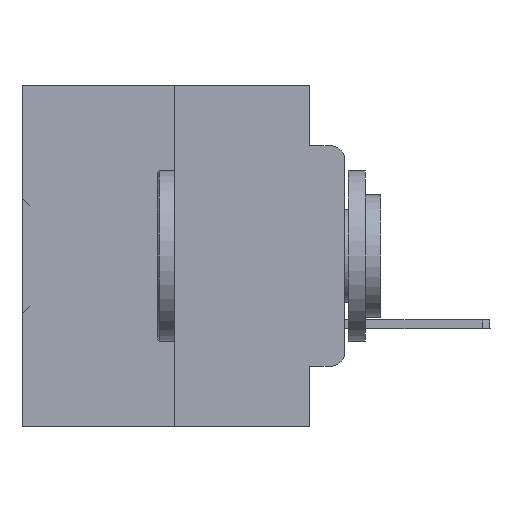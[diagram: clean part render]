
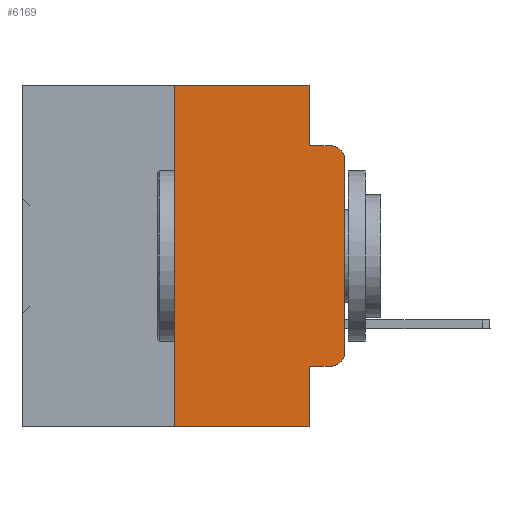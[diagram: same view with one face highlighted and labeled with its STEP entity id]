
A CAD part, left-side view. The second image highlights one B-rep face of the part: STEP entity #6169.
In plain terms, the highlighted planar face has unit normal (-1, 0, 0).
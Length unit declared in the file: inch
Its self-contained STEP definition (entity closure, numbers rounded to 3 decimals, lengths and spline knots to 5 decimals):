
#433 = EDGE_CURVE ( 'NONE', #15531, #33314, #8550, .T. ) ;
#893 = EDGE_CURVE ( 'NONE', #14730, #23608, #2235, .T. ) ;
#1037 = DIRECTION ( 'NONE',  ( -1., 0., 0. ) ) ;
#1055 = CARTESIAN_POINT ( 'NONE',  ( 0., 0.02, -0.4115 ) ) ;
#1373 = EDGE_CURVE ( 'NONE', #15531, #6546, #26735, .T. ) ;
#2119 = DIRECTION ( 'NONE',  ( 0., 0., -1. ) ) ;
#2175 = EDGE_CURVE ( 'NONE', #32285, #13042, #3916, .T. ) ;
#2187 = CIRCLE ( 'NONE', #2769, 0.02 ) ;
#2235 = LINE ( 'NONE', #36081, #32246 ) ;
#2302 = EDGE_CURVE ( 'NONE', #16048, #32285, #34897, .T. ) ;
#2687 = CARTESIAN_POINT ( 'NONE',  ( 0., 0.02, -0.0885 ) ) ;
#2769 = AXIS2_PLACEMENT_3D ( 'NONE', #16671, #11611, #9258 ) ;
#3916 = CIRCLE ( 'NONE', #25714, 0.02 ) ;
#4508 = ORIENTED_EDGE ( 'NONE', *, *, #27720, .T. ) ;
#6000 = ORIENTED_EDGE ( 'NONE', *, *, #433, .F. ) ;
#6111 = ORIENTED_EDGE ( 'NONE', *, *, #1373, .T. ) ;
#6169 = ADVANCED_FACE ( 'NONE', ( #13378 ), #34118, .F. ) ;
#6546 = VERTEX_POINT ( 'NONE', #1055 ) ;
#8550 = LINE ( 'NONE', #13846, #23174 ) ;
#8713 = VECTOR ( 'NONE', #26319, 39.37008 ) ;
#9154 = CARTESIAN_POINT ( 'NONE',  ( 0., 0., -0.1085 ) ) ;
#9258 = DIRECTION ( 'NONE',  ( 0., 0., -1. ) ) ;
#9400 = VERTEX_POINT ( 'NONE', #15428 ) ;
#9628 = ORIENTED_EDGE ( 'NONE', *, *, #30023, .F. ) ;
#10316 = CARTESIAN_POINT ( 'NONE',  ( 0., 0.051, 0. ) ) ;
#11221 = CARTESIAN_POINT ( 'NONE',  ( 0., 0., 0. ) ) ;
#11611 = DIRECTION ( 'NONE',  ( -1., 0., 0. ) ) ;
#12329 = LINE ( 'NONE', #17293, #8713 ) ;
#13042 = VERTEX_POINT ( 'NONE', #2687 ) ;
#13378 = FACE_OUTER_BOUND ( 'NONE', #24268, .T. ) ;
#13846 = CARTESIAN_POINT ( 'NONE',  ( 0., 0.051, 0. ) ) ;
#14137 = DIRECTION ( 'NONE',  ( 0., 0., 1. ) ) ;
#14222 = ORIENTED_EDGE ( 'NONE', *, *, #893, .F. ) ;
#14730 = VERTEX_POINT ( 'NONE', #10316 ) ;
#15428 = CARTESIAN_POINT ( 'NONE',  ( 0., 0.25, 0. ) ) ;
#15531 = VERTEX_POINT ( 'NONE', #16710 ) ;
#16048 = VERTEX_POINT ( 'NONE', #23652 ) ;
#16671 = CARTESIAN_POINT ( 'NONE',  ( 0., 0.02, -0.3915 ) ) ;
#16710 = CARTESIAN_POINT ( 'NONE',  ( 0., 0.051, -0.4115 ) ) ;
#16753 = VECTOR ( 'NONE', #24109, 39.37008 ) ;
#17137 = DIRECTION ( 'NONE',  ( 0., -1., 0. ) ) ;
#17293 = CARTESIAN_POINT ( 'NONE',  ( 0., 0.051, -0.0885 ) ) ;
#17766 = ORIENTED_EDGE ( 'NONE', *, *, #2175, .T. ) ;
#17842 = ORIENTED_EDGE ( 'NONE', *, *, #27552, .T. ) ;
#18641 = DIRECTION ( 'NONE',  ( 0., 0., -1. ) ) ;
#20095 = LINE ( 'NONE', #22673, #22781 ) ;
#21572 = CARTESIAN_POINT ( 'NONE',  ( 0., 0.02, -0.1085 ) ) ;
#21641 = CARTESIAN_POINT ( 'NONE',  ( 0., 0.051, -0.4115 ) ) ;
#22141 = CARTESIAN_POINT ( 'NONE',  ( 0., 0.473, 0. ) ) ;
#22370 = DIRECTION ( 'NONE',  ( 0., 0., -1. ) ) ;
#22514 = CARTESIAN_POINT ( 'NONE',  ( 0., 0.051, -0.0885 ) ) ;
#22673 = CARTESIAN_POINT ( 'NONE',  ( 0., 0.25, 0. ) ) ;
#22781 = VECTOR ( 'NONE', #14137, 39.37008 ) ;
#23174 = VECTOR ( 'NONE', #22370, 39.37008 ) ;
#23608 = VERTEX_POINT ( 'NONE', #22514 ) ;
#23611 = EDGE_CURVE ( 'NONE', #9400, #14730, #36912, .T. ) ;
#23652 = CARTESIAN_POINT ( 'NONE',  ( 0., 0., -0.3915 ) ) ;
#24109 = DIRECTION ( 'NONE',  ( 0., -1., 0. ) ) ;
#24268 = EDGE_LOOP ( 'NONE', ( #30682, #17766, #32520, #14222, #26346, #9628, #4508, #6000, #6111, #17842 ) ) ;
#24500 = LINE ( 'NONE', #35268, #16753 ) ;
#24695 = VERTEX_POINT ( 'NONE', #25499 ) ;
#25499 = CARTESIAN_POINT ( 'NONE',  ( 0., 0.25, -0.5 ) ) ;
#25714 = AXIS2_PLACEMENT_3D ( 'NONE', #21572, #1037, #2119 ) ;
#26319 = DIRECTION ( 'NONE',  ( 0., -1., 0. ) ) ;
#26346 = ORIENTED_EDGE ( 'NONE', *, *, #23611, .F. ) ;
#26719 = AXIS2_PLACEMENT_3D ( 'NONE', #22141, #28290, #31216 ) ;
#26735 = LINE ( 'NONE', #21641, #33595 ) ;
#27159 = VECTOR ( 'NONE', #35375, 39.37008 ) ;
#27524 = DIRECTION ( 'NONE',  ( 0., -1., 0. ) ) ;
#27552 = EDGE_CURVE ( 'NONE', #6546, #16048, #2187, .T. ) ;
#27720 = EDGE_CURVE ( 'NONE', #24695, #33314, #24500, .T. ) ;
#28130 = CARTESIAN_POINT ( 'NONE',  ( 0., 0.473, 0. ) ) ;
#28290 = DIRECTION ( 'NONE',  ( 1., 0., 0. ) ) ;
#29148 = VECTOR ( 'NONE', #17137, 39.37008 ) ;
#30023 = EDGE_CURVE ( 'NONE', #24695, #9400, #20095, .T. ) ;
#30682 = ORIENTED_EDGE ( 'NONE', *, *, #2302, .T. ) ;
#31216 = DIRECTION ( 'NONE',  ( 0., 0., -1. ) ) ;
#32246 = VECTOR ( 'NONE', #18641, 39.37008 ) ;
#32285 = VERTEX_POINT ( 'NONE', #9154 ) ;
#32520 = ORIENTED_EDGE ( 'NONE', *, *, #32688, .F. ) ;
#32688 = EDGE_CURVE ( 'NONE', #23608, #13042, #12329, .T. ) ;
#33314 = VERTEX_POINT ( 'NONE', #34707 ) ;
#33595 = VECTOR ( 'NONE', #27524, 39.37008 ) ;
#34118 = PLANE ( 'NONE',  #26719 ) ;
#34707 = CARTESIAN_POINT ( 'NONE',  ( 0., 0.051, -0.5 ) ) ;
#34897 = LINE ( 'NONE', #11221, #27159 ) ;
#35268 = CARTESIAN_POINT ( 'NONE',  ( 0., 0.473, -0.5 ) ) ;
#35375 = DIRECTION ( 'NONE',  ( 0., 0., 1. ) ) ;
#36081 = CARTESIAN_POINT ( 'NONE',  ( 0., 0.051, 0. ) ) ;
#36912 = LINE ( 'NONE', #28130, #29148 ) ;
